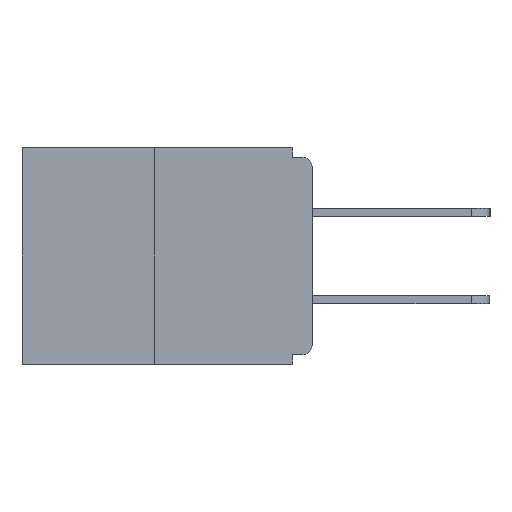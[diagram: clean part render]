
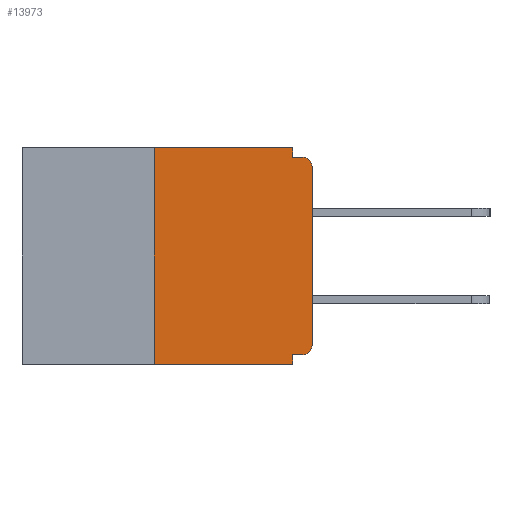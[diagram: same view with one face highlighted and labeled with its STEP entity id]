
A CAD part, left-side view. The second image highlights one B-rep face of the part: STEP entity #13973.
In plain terms, the highlighted planar face has unit normal (-1, 0, 0).
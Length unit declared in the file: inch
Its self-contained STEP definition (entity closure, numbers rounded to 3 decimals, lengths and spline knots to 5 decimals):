
#131 = LINE ( 'NONE', #10229, #12628 ) ;
#808 = CARTESIAN_POINT ( 'NONE',  ( 0., 0.25, 0. ) ) ;
#896 = DIRECTION ( 'NONE',  ( 0., 0., 1. ) ) ;
#1127 = PLANE ( 'NONE',  #19468 ) ;
#1763 = ORIENTED_EDGE ( 'NONE', *, *, #27413, .T. ) ;
#1884 = EDGE_CURVE ( 'NONE', #4540, #15524, #22335, .T. ) ;
#2088 = LINE ( 'NONE', #13263, #2771 ) ;
#2292 = CIRCLE ( 'NONE', #22226, 0.015 ) ;
#2321 = ORIENTED_EDGE ( 'NONE', *, *, #13817, .T. ) ;
#2646 = VERTEX_POINT ( 'NONE', #18001 ) ;
#2771 = VECTOR ( 'NONE', #4346, 39.37008 ) ;
#2973 = ORIENTED_EDGE ( 'NONE', *, *, #22214, .T. ) ;
#3141 = FACE_OUTER_BOUND ( 'NONE', #10729, .T. ) ;
#3350 = CARTESIAN_POINT ( 'NONE',  ( 0., 0.46, 0. ) ) ;
#3745 = VERTEX_POINT ( 'NONE', #18058 ) ;
#4341 = CARTESIAN_POINT ( 'NONE',  ( 0., 0.015, -0.03 ) ) ;
#4346 = DIRECTION ( 'NONE',  ( 0., 0., -1. ) ) ;
#4540 = VERTEX_POINT ( 'NONE', #18358 ) ;
#5329 = EDGE_CURVE ( 'NONE', #25835, #4540, #2088, .T. ) ;
#5597 = DIRECTION ( 'NONE',  ( 0., -1., 0. ) ) ;
#5637 = CARTESIAN_POINT ( 'NONE',  ( 0., 0.25, -0.343 ) ) ;
#6312 = CARTESIAN_POINT ( 'NONE',  ( 0., 0.46, -0.343 ) ) ;
#6656 = VERTEX_POINT ( 'NONE', #18519 ) ;
#7049 = DIRECTION ( 'NONE',  ( 0., -1., 0. ) ) ;
#7197 = VERTEX_POINT ( 'NONE', #5637 ) ;
#7553 = CARTESIAN_POINT ( 'NONE',  ( 0., 0., -0.313 ) ) ;
#7653 = CARTESIAN_POINT ( 'NONE',  ( 0., 0.015, -0.328 ) ) ;
#7828 = DIRECTION ( 'NONE',  ( 1., 0., 0. ) ) ;
#8239 = ORIENTED_EDGE ( 'NONE', *, *, #8253, .F. ) ;
#8253 = EDGE_CURVE ( 'NONE', #2646, #8335, #15432, .T. ) ;
#8294 = VECTOR ( 'NONE', #5597, 39.37008 ) ;
#8335 = VERTEX_POINT ( 'NONE', #8771 ) ;
#8348 = DIRECTION ( 'NONE',  ( 0., 0., -1. ) ) ;
#8771 = CARTESIAN_POINT ( 'NONE',  ( 0., 0.031, -0.343 ) ) ;
#10229 = CARTESIAN_POINT ( 'NONE',  ( 0., 0., 0. ) ) ;
#10379 = EDGE_CURVE ( 'NONE', #7197, #6656, #14291, .T. ) ;
#10579 = DIRECTION ( 'NONE',  ( 0., -1., 0. ) ) ;
#10729 = EDGE_LOOP ( 'NONE', ( #14110, #26888, #1763, #8239, #14309, #16783, #2973, #2321, #20531, #23589 ) ) ;
#11290 = DIRECTION ( 'NONE',  ( 0., 0., -1. ) ) ;
#12527 = CIRCLE ( 'NONE', #26462, 0.015 ) ;
#12628 = VECTOR ( 'NONE', #16874, 39.37008 ) ;
#12830 = CARTESIAN_POINT ( 'NONE',  ( 0., 0., -0.328 ) ) ;
#12904 = CARTESIAN_POINT ( 'NONE',  ( 0., 0.015, -0.313 ) ) ;
#13166 = DIRECTION ( 'NONE',  ( 0., 0., -1. ) ) ;
#13263 = CARTESIAN_POINT ( 'NONE',  ( 0., 0.031, 0. ) ) ;
#13817 = EDGE_CURVE ( 'NONE', #3745, #15524, #12527, .T. ) ;
#13973 = ADVANCED_FACE ( 'NONE', ( #3141 ), #1127, .F. ) ;
#14110 = ORIENTED_EDGE ( 'NONE', *, *, #26136, .F. ) ;
#14291 = LINE ( 'NONE', #808, #24300 ) ;
#14309 = ORIENTED_EDGE ( 'NONE', *, *, #14373, .F. ) ;
#14373 = EDGE_CURVE ( 'NONE', #25051, #2646, #27288, .T. ) ;
#15432 = LINE ( 'NONE', #15587, #20967 ) ;
#15524 = VERTEX_POINT ( 'NONE', #24915 ) ;
#15587 = CARTESIAN_POINT ( 'NONE',  ( 0., 0.031, -0.343 ) ) ;
#15751 = VECTOR ( 'NONE', #7049, 39.37008 ) ;
#16260 = VECTOR ( 'NONE', #21391, 39.37008 ) ;
#16783 = ORIENTED_EDGE ( 'NONE', *, *, #27488, .T. ) ;
#16848 = VERTEX_POINT ( 'NONE', #7553 ) ;
#16874 = DIRECTION ( 'NONE',  ( 0., 0., 1. ) ) ;
#18001 = CARTESIAN_POINT ( 'NONE',  ( 0., 0.031, -0.328 ) ) ;
#18058 = CARTESIAN_POINT ( 'NONE',  ( 0., 0., -0.03 ) ) ;
#18358 = CARTESIAN_POINT ( 'NONE',  ( 0., 0.031, -0.015 ) ) ;
#18519 = CARTESIAN_POINT ( 'NONE',  ( 0., 0.25, 0. ) ) ;
#18523 = DIRECTION ( 'NONE',  ( 0., 0., -1. ) ) ;
#19468 = AXIS2_PLACEMENT_3D ( 'NONE', #3350, #7828, #18523 ) ;
#19568 = CARTESIAN_POINT ( 'NONE',  ( 0., 0.031, 0. ) ) ;
#19577 = LINE ( 'NONE', #6312, #25792 ) ;
#20444 = CARTESIAN_POINT ( 'NONE',  ( 0., 0., -0.015 ) ) ;
#20531 = ORIENTED_EDGE ( 'NONE', *, *, #1884, .F. ) ;
#20967 = VECTOR ( 'NONE', #11290, 39.37008 ) ;
#21391 = DIRECTION ( 'NONE',  ( 0., 1., 0. ) ) ;
#21552 = DIRECTION ( 'NONE',  ( -1., 0., 0. ) ) ;
#22214 = EDGE_CURVE ( 'NONE', #16848, #3745, #131, .T. ) ;
#22226 = AXIS2_PLACEMENT_3D ( 'NONE', #12904, #21552, #8348 ) ;
#22335 = LINE ( 'NONE', #20444, #15751 ) ;
#22432 = LINE ( 'NONE', #23063, #8294 ) ;
#23063 = CARTESIAN_POINT ( 'NONE',  ( 0., 0.46, 0. ) ) ;
#23589 = ORIENTED_EDGE ( 'NONE', *, *, #5329, .F. ) ;
#24222 = DIRECTION ( 'NONE',  ( -1., 0., 0. ) ) ;
#24300 = VECTOR ( 'NONE', #896, 39.37008 ) ;
#24915 = CARTESIAN_POINT ( 'NONE',  ( 0., 0.015, -0.015 ) ) ;
#25051 = VERTEX_POINT ( 'NONE', #7653 ) ;
#25792 = VECTOR ( 'NONE', #10579, 39.37008 ) ;
#25835 = VERTEX_POINT ( 'NONE', #19568 ) ;
#26136 = EDGE_CURVE ( 'NONE', #6656, #25835, #22432, .T. ) ;
#26462 = AXIS2_PLACEMENT_3D ( 'NONE', #4341, #24222, #13166 ) ;
#26888 = ORIENTED_EDGE ( 'NONE', *, *, #10379, .F. ) ;
#27288 = LINE ( 'NONE', #12830, #16260 ) ;
#27413 = EDGE_CURVE ( 'NONE', #7197, #8335, #19577, .T. ) ;
#27488 = EDGE_CURVE ( 'NONE', #25051, #16848, #2292, .T. ) ;
